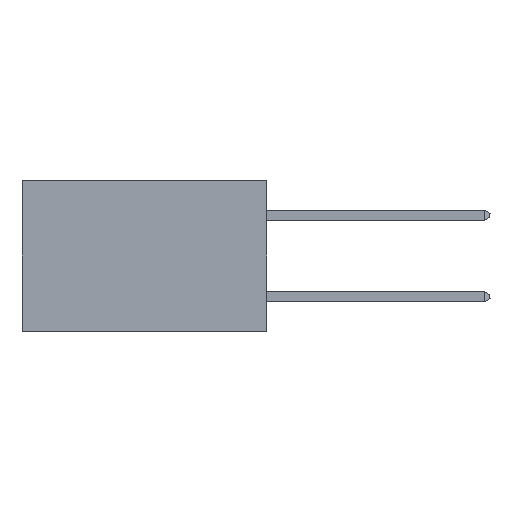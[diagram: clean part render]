
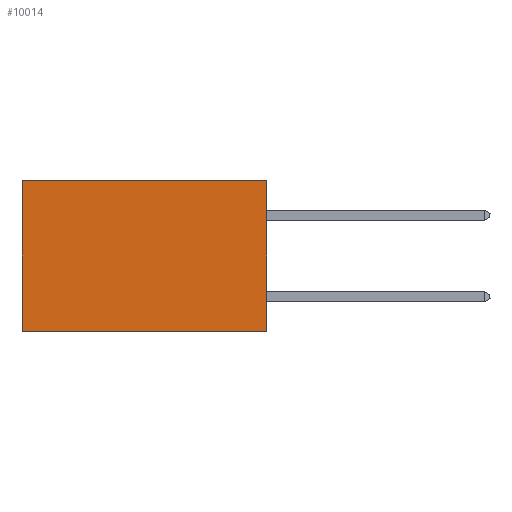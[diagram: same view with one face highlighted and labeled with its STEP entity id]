
A CAD part, left-side view. The second image highlights one B-rep face of the part: STEP entity #10014.
In plain terms, the highlighted planar face has unit normal (-1, 0, 0).
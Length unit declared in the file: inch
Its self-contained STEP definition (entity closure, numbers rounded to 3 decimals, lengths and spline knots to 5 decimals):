
#696 = CARTESIAN_POINT ( 'NONE',  ( 0.2875, 0.6, 0. ) ) ;
#802 = DIRECTION ( 'NONE',  ( 0., 0., -1. ) ) ;
#1257 = LINE ( 'NONE', #2274, #22620 ) ;
#2274 = CARTESIAN_POINT ( 'NONE',  ( 0.2875, 0., -0.37 ) ) ;
#2754 = CARTESIAN_POINT ( 'NONE',  ( 0.2875, 0., 0. ) ) ;
#3812 = LINE ( 'NONE', #15626, #18319 ) ;
#5319 = DIRECTION ( 'NONE',  ( 0., 0., -1. ) ) ;
#5364 = VERTEX_POINT ( 'NONE', #23350 ) ;
#6298 = EDGE_CURVE ( 'NONE', #19025, #23213, #16731, .T. ) ;
#6533 = ORIENTED_EDGE ( 'NONE', *, *, #20091, .T. ) ;
#7957 = EDGE_LOOP ( 'NONE', ( #17872, #7980, #15791, #6533 ) ) ;
#7980 = ORIENTED_EDGE ( 'NONE', *, *, #15809, .F. ) ;
#8168 = DIRECTION ( 'NONE',  ( 0., 1., 0. ) ) ;
#9396 = VERTEX_POINT ( 'NONE', #10485 ) ;
#10014 = ADVANCED_FACE ( 'NONE', ( #21764 ), #17531, .F. ) ;
#10485 = CARTESIAN_POINT ( 'NONE',  ( 0.2875, 0., -0.37 ) ) ;
#15237 = DIRECTION ( 'NONE',  ( 0., 0., -1. ) ) ;
#15314 = VECTOR ( 'NONE', #15237, 39.37008 ) ;
#15626 = CARTESIAN_POINT ( 'NONE',  ( 0.2875, 0., 0. ) ) ;
#15791 = ORIENTED_EDGE ( 'NONE', *, *, #21931, .F. ) ;
#15809 = EDGE_CURVE ( 'NONE', #9396, #23213, #1257, .T. ) ;
#16436 = DIRECTION ( 'NONE',  ( 0., 1., 0. ) ) ;
#16731 = LINE ( 'NONE', #696, #15314 ) ;
#17285 = CARTESIAN_POINT ( 'NONE',  ( 0.2875, 0., 0. ) ) ;
#17531 = PLANE ( 'NONE',  #23074 ) ;
#17577 = CARTESIAN_POINT ( 'NONE',  ( 0.2875, 0.6, 0. ) ) ;
#17872 = ORIENTED_EDGE ( 'NONE', *, *, #6298, .T. ) ;
#18319 = VECTOR ( 'NONE', #8168, 39.37008 ) ;
#19025 = VERTEX_POINT ( 'NONE', #17577 ) ;
#20091 = EDGE_CURVE ( 'NONE', #5364, #19025, #3812, .T. ) ;
#20270 = VECTOR ( 'NONE', #5319, 39.37008 ) ;
#20586 = LINE ( 'NONE', #2754, #20270 ) ;
#21061 = DIRECTION ( 'NONE',  ( 1., 0., 0. ) ) ;
#21725 = CARTESIAN_POINT ( 'NONE',  ( 0.2875, 0.6, -0.37 ) ) ;
#21764 = FACE_OUTER_BOUND ( 'NONE', #7957, .T. ) ;
#21931 = EDGE_CURVE ( 'NONE', #5364, #9396, #20586, .T. ) ;
#22620 = VECTOR ( 'NONE', #16436, 39.37008 ) ;
#23074 = AXIS2_PLACEMENT_3D ( 'NONE', #17285, #21061, #802 ) ;
#23213 = VERTEX_POINT ( 'NONE', #21725 ) ;
#23350 = CARTESIAN_POINT ( 'NONE',  ( 0.2875, 0., 0. ) ) ;
